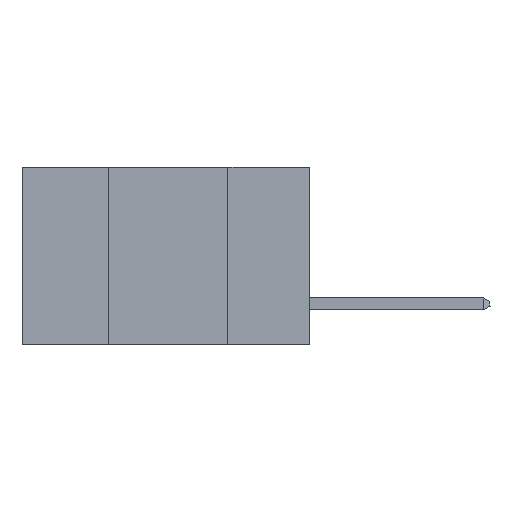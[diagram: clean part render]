
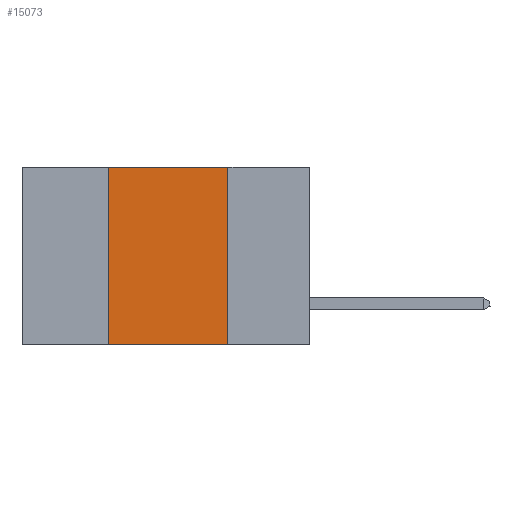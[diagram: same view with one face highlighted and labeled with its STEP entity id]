
A CAD part, left-side view. The second image highlights one B-rep face of the part: STEP entity #15073.
In plain terms, the highlighted planar face has unit normal (-1, 0, 0).
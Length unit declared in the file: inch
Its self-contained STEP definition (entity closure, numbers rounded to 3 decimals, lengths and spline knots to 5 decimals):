
#524 = ORIENTED_EDGE ( 'NONE', *, *, #11223, .F. ) ;
#654 = ORIENTED_EDGE ( 'NONE', *, *, #17960, .F. ) ;
#777 = EDGE_CURVE ( 'NONE', #6131, #19010, #13502, .T. ) ;
#908 = CARTESIAN_POINT ( 'NONE',  ( 0., 0.42, 0. ) ) ;
#3171 = CARTESIAN_POINT ( 'NONE',  ( 0., 0.42, -0.37 ) ) ;
#3262 = VERTEX_POINT ( 'NONE', #10196 ) ;
#3741 = PLANE ( 'NONE',  #6714 ) ;
#3975 = VECTOR ( 'NONE', #10627, 39.37008 ) ;
#4060 = CARTESIAN_POINT ( 'NONE',  ( 0., 0.6, -0.37 ) ) ;
#5241 = CARTESIAN_POINT ( 'NONE',  ( 0., 0.6, 0. ) ) ;
#5585 = CARTESIAN_POINT ( 'NONE',  ( 0., 0.17, 0. ) ) ;
#5605 = DIRECTION ( 'NONE',  ( 1., 0., 0. ) ) ;
#5859 = CARTESIAN_POINT ( 'NONE',  ( 0., 0.42, 0. ) ) ;
#6131 = VERTEX_POINT ( 'NONE', #5859 ) ;
#6147 = DIRECTION ( 'NONE',  ( 0., -1., 0. ) ) ;
#6531 = ORIENTED_EDGE ( 'NONE', *, *, #20231, .T. ) ;
#6714 = AXIS2_PLACEMENT_3D ( 'NONE', #7600, #5605, #13264 ) ;
#7600 = CARTESIAN_POINT ( 'NONE',  ( 0., 0.6, 0. ) ) ;
#8103 = DIRECTION ( 'NONE',  ( 0., 0., 1. ) ) ;
#8854 = ORIENTED_EDGE ( 'NONE', *, *, #777, .F. ) ;
#8932 = LINE ( 'NONE', #4060, #18711 ) ;
#10196 = CARTESIAN_POINT ( 'NONE',  ( 0., 0.17, -0.37 ) ) ;
#10627 = DIRECTION ( 'NONE',  ( 0., -1., 0. ) ) ;
#11223 = EDGE_CURVE ( 'NONE', #19010, #3262, #20957, .T. ) ;
#12525 = LINE ( 'NONE', #908, #13100 ) ;
#13100 = VECTOR ( 'NONE', #8103, 39.37008 ) ;
#13264 = DIRECTION ( 'NONE',  ( 0., 0., -1. ) ) ;
#13502 = LINE ( 'NONE', #5241, #3975 ) ;
#15073 = ADVANCED_FACE ( 'NONE', ( #22373 ), #3741, .F. ) ;
#16990 = VECTOR ( 'NONE', #20239, 39.37008 ) ;
#17960 = EDGE_CURVE ( 'NONE', #21015, #6131, #12525, .T. ) ;
#18711 = VECTOR ( 'NONE', #6147, 39.37008 ) ;
#19010 = VERTEX_POINT ( 'NONE', #23049 ) ;
#19725 = EDGE_LOOP ( 'NONE', ( #524, #8854, #654, #6531 ) ) ;
#20231 = EDGE_CURVE ( 'NONE', #21015, #3262, #8932, .T. ) ;
#20239 = DIRECTION ( 'NONE',  ( 0., 0., -1. ) ) ;
#20957 = LINE ( 'NONE', #5585, #16990 ) ;
#21015 = VERTEX_POINT ( 'NONE', #3171 ) ;
#22373 = FACE_OUTER_BOUND ( 'NONE', #19725, .T. ) ;
#23049 = CARTESIAN_POINT ( 'NONE',  ( 0., 0.17, 0. ) ) ;
